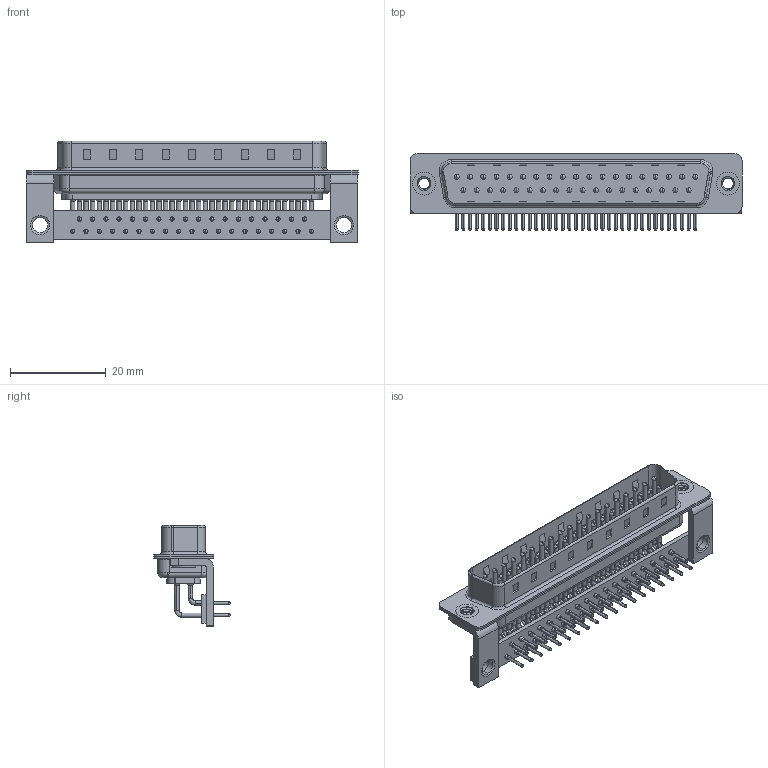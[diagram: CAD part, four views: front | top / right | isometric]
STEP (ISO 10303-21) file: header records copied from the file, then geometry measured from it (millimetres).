
FILE_DESCRIPTION (( 'STEP AP203' ), '1' );
FILE_NAME ('629-M37-640-WN4.STEP', '2018-09-25T22:40:24', ( '' ), ( '' ), 'SwSTEP 2.0', 'SolidWorks 2016', '' );
FILE_SCHEMA (( 'CONFIG_CONTROL_DESIGN' ));
Length unit declared in the file: millimetre
Products named in the file (9): 629M 4-40 Threaded Rivet_Stabilizer; 629M Stabilizer Bracket; 629M Stabilizer Board_37 Contacts; 629-M37-640-WN4; 629M Shell Rear_37 Contacts; 629M Housing_37 Contacts; 629M Contact Row 1; 629M Shell Front_37 Contacts; 629M Contact Row 2
Assembly tree (45 placements, depth 2):
  629-M37-640-WN4
    629M Housing_37 Contacts
    629M Shell Front_37 Contacts
    629M Shell Rear_37 Contacts
    629M Contact Row 1  x19
    629M Contact Row 2  x18
    629M 4-40 Threaded Rivet_Stabilizer  x2
    629M Stabilizer Bracket  x2
    629M Stabilizer Board_37 Contacts
Bounding box: 69.4 x 16 x 21.3 mm (x, y, z)
Volume: 4693.5 mm3; surface area: 12232.4 mm2
Topology: 45 solids, 45 shells, 4606 faces, 12919 edges, 8414 vertices
Faces by surface type: plane 2597, cylinder 1569, bspline 228, cone 156, torus 56
Entity records: 34138 total; most frequent: CARTESIAN_POINT 6868, DIRECTION 5583, ORIENTED_EDGE 5040, EDGE_CURVE 2520, AXIS2_PLACEMENT_3D 2090, VERTEX_POINT 1640, VECTOR 1403, LINE 1403
